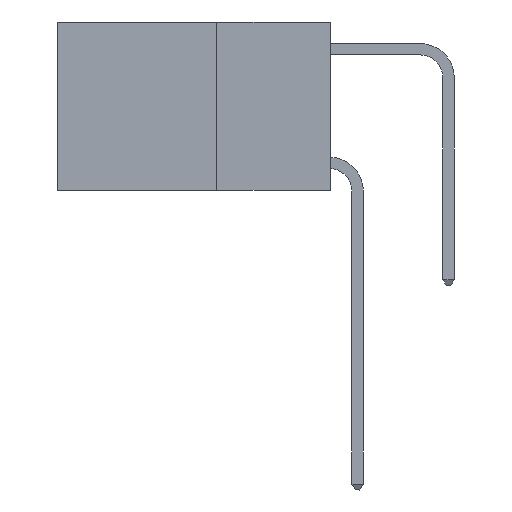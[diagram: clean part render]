
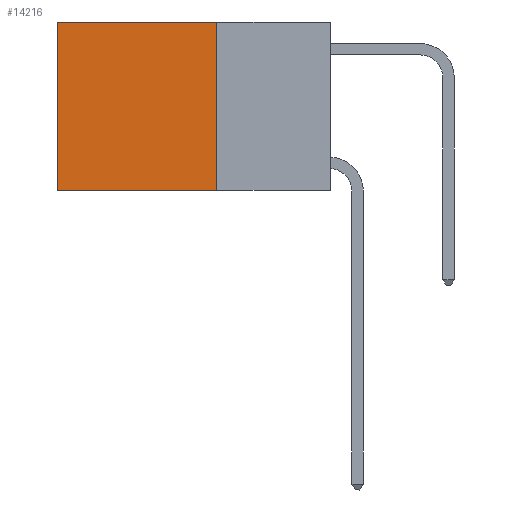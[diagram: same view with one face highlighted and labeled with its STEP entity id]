
A CAD part, left-side view. The second image highlights one B-rep face of the part: STEP entity #14216.
In plain terms, the highlighted planar face has unit normal (-1, 0, 0).
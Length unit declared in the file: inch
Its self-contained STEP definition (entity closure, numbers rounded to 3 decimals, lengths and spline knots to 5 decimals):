
#1296 = ORIENTED_EDGE ( 'NONE', *, *, #5058, .F. ) ;
#2873 = VERTEX_POINT ( 'NONE', #8861 ) ;
#3360 = ORIENTED_EDGE ( 'NONE', *, *, #12412, .F. ) ;
#3506 = CARTESIAN_POINT ( 'NONE',  ( 0.2625, 0.25, 0. ) ) ;
#3732 = PLANE ( 'NONE',  #5537 ) ;
#3927 = EDGE_CURVE ( 'NONE', #11575, #4556, #6020, .T. ) ;
#3965 = CARTESIAN_POINT ( 'NONE',  ( 0.2625, 0.6, -0.37 ) ) ;
#4067 = CARTESIAN_POINT ( 'NONE',  ( 0.2625, 0.25, -0.37 ) ) ;
#4556 = VERTEX_POINT ( 'NONE', #3965 ) ;
#5058 = EDGE_CURVE ( 'NONE', #2873, #4556, #10223, .T. ) ;
#5537 = AXIS2_PLACEMENT_3D ( 'NONE', #3506, #9890, #9811 ) ;
#6020 = LINE ( 'NONE', #9926, #11467 ) ;
#7227 = EDGE_CURVE ( 'NONE', #8391, #11575, #8740, .T. ) ;
#7615 = VECTOR ( 'NONE', #14580, 39.37008 ) ;
#8391 = VERTEX_POINT ( 'NONE', #14397 ) ;
#8453 = CARTESIAN_POINT ( 'NONE',  ( 0.2625, 0.25, 0. ) ) ;
#8686 = LINE ( 'NONE', #8453, #7615 ) ;
#8740 = LINE ( 'NONE', #9638, #12519 ) ;
#8861 = CARTESIAN_POINT ( 'NONE',  ( 0.2625, 0.25, -0.37 ) ) ;
#9007 = DIRECTION ( 'NONE',  ( 0., 1., 0. ) ) ;
#9638 = CARTESIAN_POINT ( 'NONE',  ( 0.2625, 0.25, 0. ) ) ;
#9687 = ORIENTED_EDGE ( 'NONE', *, *, #3927, .T. ) ;
#9811 = DIRECTION ( 'NONE',  ( 0., 0., -1. ) ) ;
#9890 = DIRECTION ( 'NONE',  ( 1., 0., 0. ) ) ;
#9926 = CARTESIAN_POINT ( 'NONE',  ( 0.2625, 0.6, 0. ) ) ;
#10223 = LINE ( 'NONE', #4067, #14319 ) ;
#11097 = ORIENTED_EDGE ( 'NONE', *, *, #7227, .T. ) ;
#11467 = VECTOR ( 'NONE', #12277, 39.37008 ) ;
#11575 = VERTEX_POINT ( 'NONE', #15566 ) ;
#12277 = DIRECTION ( 'NONE',  ( 0., 0., -1. ) ) ;
#12319 = FACE_OUTER_BOUND ( 'NONE', #15176, .T. ) ;
#12412 = EDGE_CURVE ( 'NONE', #8391, #2873, #8686, .T. ) ;
#12519 = VECTOR ( 'NONE', #14559, 39.37008 ) ;
#14216 = ADVANCED_FACE ( 'NONE', ( #12319 ), #3732, .F. ) ;
#14319 = VECTOR ( 'NONE', #9007, 39.37008 ) ;
#14397 = CARTESIAN_POINT ( 'NONE',  ( 0.2625, 0.25, 0. ) ) ;
#14559 = DIRECTION ( 'NONE',  ( 0., 1., 0. ) ) ;
#14580 = DIRECTION ( 'NONE',  ( 0., 0., -1. ) ) ;
#15176 = EDGE_LOOP ( 'NONE', ( #9687, #1296, #3360, #11097 ) ) ;
#15566 = CARTESIAN_POINT ( 'NONE',  ( 0.2625, 0.6, 0. ) ) ;
